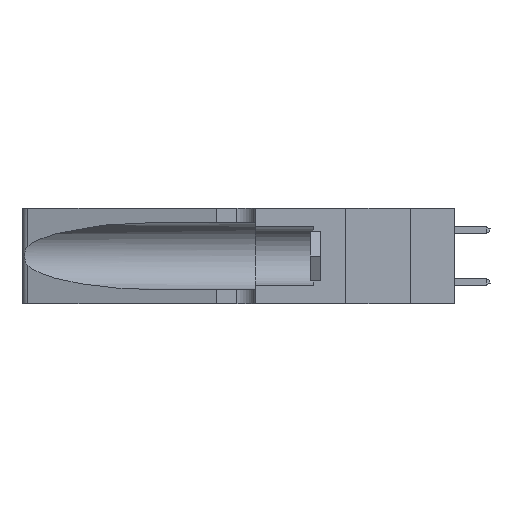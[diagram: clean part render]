
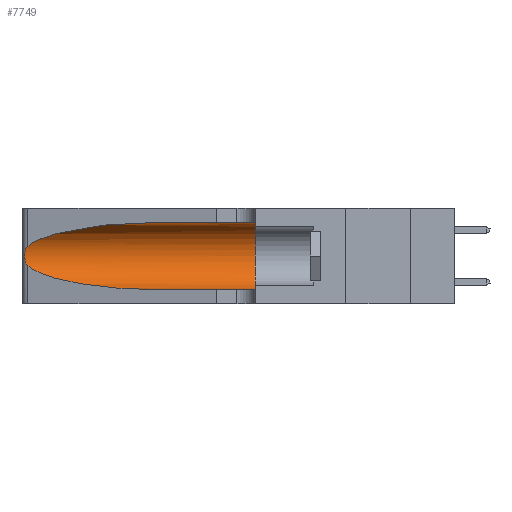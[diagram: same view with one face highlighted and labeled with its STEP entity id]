
A CAD part, left-side view. The second image highlights one B-rep face of the part: STEP entity #7749.
In plain terms, the highlighted cylindrical face has radius 3.308 mm (diameter 6.617 mm), a partial arc.
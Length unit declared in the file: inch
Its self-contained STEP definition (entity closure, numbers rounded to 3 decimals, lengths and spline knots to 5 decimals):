
#197 = VERTEX_POINT ( 'NONE', #15495 ) ;
#858 = DIRECTION ( 'NONE',  ( 0., -1., 0. ) ) ;
#1069 = CARTESIAN_POINT ( 'NONE',  ( 0.25639, 1.23184, 0.21858 ) ) ;
#1084 = CARTESIAN_POINT ( 'NONE',  ( 0.1305, 0.72297, 0.05475 ) ) ;
#1144 = DIRECTION ( 'NONE',  ( 0., -1., 0. ) ) ;
#1846 = DIRECTION ( 'NONE',  ( 0., -1., 0. ) ) ;
#1872 = CARTESIAN_POINT ( 'NONE',  ( 0.1305, 0.72297, 0.05475 ) ) ;
#2497 = CARTESIAN_POINT ( 'NONE',  ( 0.18966, 0.96281, 0.31525 ) ) ;
#2780 = CARTESIAN_POINT ( 'NONE',  ( 0.26075, 1.23896, 0.178 ) ) ;
#2944 = CARTESIAN_POINT ( 'NONE',  ( 0.18966, 0.96281, 0.05475 ) ) ;
#3312 = DIRECTION ( 'NONE',  ( 0., 0., 1. ) ) ;
#3325 = EDGE_CURVE ( 'NONE', #15521, #20634, #3448, .T. ) ;
#3332 = CARTESIAN_POINT ( 'NONE',  ( 0.1305, 0.35, 0.185 ) ) ;
#3448 = LINE ( 'NONE', #12206, #10183 ) ;
#3532 = EDGE_CURVE ( 'NONE', #15521, #4470, #17948, .T. ) ;
#3936 = CIRCLE ( 'NONE', #11695, 0.13025 ) ;
#4148 = CARTESIAN_POINT ( 'NONE',  ( 0.2373, 1.15595, 0.28018 ) ) ;
#4470 = VERTEX_POINT ( 'NONE', #4633 ) ;
#4633 = CARTESIAN_POINT ( 'NONE',  ( 0.25487, 1.22718, 0.22369 ) ) ;
#4652 = CARTESIAN_POINT ( 'NONE',  ( 0.25787, 1.23484, 0.2124 ) ) ;
#4724 =( BOUNDED_CURVE ( )  B_SPLINE_CURVE ( 3, ( #13094, #11365, #2944, #1084 ),
 .UNSPECIFIED., .F., .F. ) 
 B_SPLINE_CURVE_WITH_KNOTS ( ( 4, 4 ),
 ( 3.44316, 4.71239 ),
 .UNSPECIFIED. ) 
 CURVE ( )  GEOMETRIC_REPRESENTATION_ITEM ( )  RATIONAL_B_SPLINE_CURVE ( ( 1., 0.87, 0.87, 1. ) ) 
 REPRESENTATION_ITEM ( '' )  );
#5353 = EDGE_CURVE ( 'NONE', #17082, #197, #19190, .T. ) ;
#5586 = AXIS2_PLACEMENT_3D ( 'NONE', #21595, #858, #21673 ) ;
#6228 = CARTESIAN_POINT ( 'NONE',  ( 0.25854, 1.2359, 0.20912 ) ) ;
#7051 = CARTESIAN_POINT ( 'NONE',  ( 0.1305, 0.35, 0.31525 ) ) ;
#7749 = ADVANCED_FACE ( 'NONE', ( #18849 ), #17226, .F. ) ;
#7887 = CARTESIAN_POINT ( 'NONE',  ( 0.25555, 1.22994, 0.2215 ) ) ;
#8042 = CARTESIAN_POINT ( 'NONE',  ( 0.1305, 1.61858, 0.05475 ) ) ;
#8305 = B_SPLINE_CURVE_WITH_KNOTS ( 'NONE', 3,
 ( #20083, #7887, #1069, #4652, #6228, #13078, #18098, #2780, #14799, #16595, #13292, #18241, #21785, #11491 ),
 .UNSPECIFIED., .F., .F.,
 ( 4, 2, 2, 2, 2, 2, 4 ),
 ( 0., 0.00027, 0.00053, 0.00107, 0.0016, 0.00187, 0.00214 ),
 .UNSPECIFIED. ) ;
#9239 = EDGE_CURVE ( 'NONE', #4470, #13188, #8305, .T. ) ;
#10183 = VECTOR ( 'NONE', #1846, 39.37008 ) ;
#10481 = DIRECTION ( 'NONE',  ( 0., 1., 0. ) ) ;
#10631 = ORIENTED_EDGE ( 'NONE', *, *, #20366, .T. ) ;
#11365 = CARTESIAN_POINT ( 'NONE',  ( 0.2373, 1.15595, 0.08982 ) ) ;
#11491 = CARTESIAN_POINT ( 'NONE',  ( 0.25487, 1.22718, 0.14631 ) ) ;
#11695 = AXIS2_PLACEMENT_3D ( 'NONE', #3332, #10481, #3312 ) ;
#11909 = EDGE_LOOP ( 'NONE', ( #21522, #20031, #10631, #22208, #15431, #12044 ) ) ;
#12044 = ORIENTED_EDGE ( 'NONE', *, *, #3325, .F. ) ;
#12206 = CARTESIAN_POINT ( 'NONE',  ( 0.1305, 1.61858, 0.31525 ) ) ;
#13078 = CARTESIAN_POINT ( 'NONE',  ( 0.26018, 1.23835, 0.19895 ) ) ;
#13094 = CARTESIAN_POINT ( 'NONE',  ( 0.25487, 1.22718, 0.14631 ) ) ;
#13188 = VERTEX_POINT ( 'NONE', #13349 ) ;
#13292 = CARTESIAN_POINT ( 'NONE',  ( 0.25789, 1.23486, 0.15765 ) ) ;
#13349 = CARTESIAN_POINT ( 'NONE',  ( 0.25487, 1.22718, 0.14631 ) ) ;
#13808 = EDGE_CURVE ( 'NONE', #20634, #197, #3936, .T. ) ;
#14498 = CARTESIAN_POINT ( 'NONE',  ( 0.25487, 1.22718, 0.22369 ) ) ;
#14799 = CARTESIAN_POINT ( 'NONE',  ( 0.26017, 1.23833, 0.17102 ) ) ;
#15431 = ORIENTED_EDGE ( 'NONE', *, *, #13808, .F. ) ;
#15495 = CARTESIAN_POINT ( 'NONE',  ( 0.1305, 0.35, 0.05475 ) ) ;
#15521 = VERTEX_POINT ( 'NONE', #18017 ) ;
#16595 = CARTESIAN_POINT ( 'NONE',  ( 0.25856, 1.23593, 0.16098 ) ) ;
#16783 = VECTOR ( 'NONE', #1144, 39.37008 ) ;
#17082 = VERTEX_POINT ( 'NONE', #1872 ) ;
#17226 = CYLINDRICAL_SURFACE ( 'NONE', #5586, 0.13025 ) ;
#17948 =( BOUNDED_CURVE ( )  B_SPLINE_CURVE ( 3, ( #19731, #2497, #4148, #14498 ),
 .UNSPECIFIED., .F., .F. ) 
 B_SPLINE_CURVE_WITH_KNOTS ( ( 4, 4 ),
 ( 1.5708, 2.84003 ),
 .UNSPECIFIED. ) 
 CURVE ( )  GEOMETRIC_REPRESENTATION_ITEM ( )  RATIONAL_B_SPLINE_CURVE ( ( 1., 0.87, 0.87, 1. ) ) 
 REPRESENTATION_ITEM ( '' )  );
#18017 = CARTESIAN_POINT ( 'NONE',  ( 0.1305, 0.72297, 0.31525 ) ) ;
#18098 = CARTESIAN_POINT ( 'NONE',  ( 0.26075, 1.23896, 0.19203 ) ) ;
#18241 = CARTESIAN_POINT ( 'NONE',  ( 0.25639, 1.23186, 0.15144 ) ) ;
#18849 = FACE_OUTER_BOUND ( 'NONE', #11909, .T. ) ;
#19190 = LINE ( 'NONE', #8042, #16783 ) ;
#19731 = CARTESIAN_POINT ( 'NONE',  ( 0.1305, 0.72297, 0.31525 ) ) ;
#20031 = ORIENTED_EDGE ( 'NONE', *, *, #9239, .T. ) ;
#20083 = CARTESIAN_POINT ( 'NONE',  ( 0.25487, 1.22718, 0.22369 ) ) ;
#20366 = EDGE_CURVE ( 'NONE', #13188, #17082, #4724, .T. ) ;
#20634 = VERTEX_POINT ( 'NONE', #7051 ) ;
#21522 = ORIENTED_EDGE ( 'NONE', *, *, #3532, .T. ) ;
#21595 = CARTESIAN_POINT ( 'NONE',  ( 0.1305, 1.61858, 0.185 ) ) ;
#21673 = DIRECTION ( 'NONE',  ( 0., 0., -1. ) ) ;
#21785 = CARTESIAN_POINT ( 'NONE',  ( 0.25555, 1.22993, 0.14849 ) ) ;
#22208 = ORIENTED_EDGE ( 'NONE', *, *, #5353, .T. ) ;
